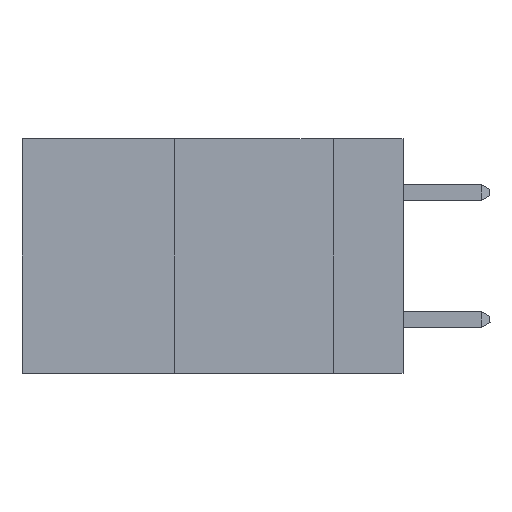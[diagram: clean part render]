
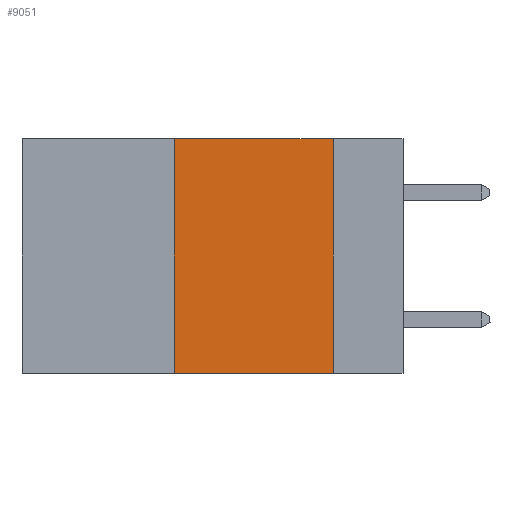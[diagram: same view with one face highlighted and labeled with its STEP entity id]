
A CAD part, left-side view. The second image highlights one B-rep face of the part: STEP entity #9051.
In plain terms, the highlighted planar face has unit normal (-1, 0, 0).
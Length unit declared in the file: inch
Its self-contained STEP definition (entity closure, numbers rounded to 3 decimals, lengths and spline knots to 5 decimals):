
#1376 = VERTEX_POINT ( 'NONE', #4658 ) ;
#2514 = CARTESIAN_POINT ( 'NONE',  ( 0., 0.6, -0.37 ) ) ;
#3719 = VERTEX_POINT ( 'NONE', #13797 ) ;
#4281 = ORIENTED_EDGE ( 'NONE', *, *, #21349, .T. ) ;
#4658 = CARTESIAN_POINT ( 'NONE',  ( 0., 0.11, -0.37 ) ) ;
#5012 = LINE ( 'NONE', #2514, #12658 ) ;
#5362 = ORIENTED_EDGE ( 'NONE', *, *, #29337, .F. ) ;
#7128 = CARTESIAN_POINT ( 'NONE',  ( 0., 0.11, 0. ) ) ;
#9051 = ADVANCED_FACE ( 'NONE', ( #9473 ), #32438, .F. ) ;
#9473 = FACE_OUTER_BOUND ( 'NONE', #40818, .T. ) ;
#10745 = LINE ( 'NONE', #16358, #35815 ) ;
#11396 = CARTESIAN_POINT ( 'NONE',  ( 0., 0.11, 0. ) ) ;
#12658 = VECTOR ( 'NONE', #22114, 39.37008 ) ;
#12799 = CARTESIAN_POINT ( 'NONE',  ( 0., 0.6, 0. ) ) ;
#13797 = CARTESIAN_POINT ( 'NONE',  ( 0., 0.36, 0. ) ) ;
#15226 = VECTOR ( 'NONE', #23618, 39.37008 ) ;
#16099 = DIRECTION ( 'NONE',  ( 1., 0., 0. ) ) ;
#16242 = LINE ( 'NONE', #7128, #15226 ) ;
#16358 = CARTESIAN_POINT ( 'NONE',  ( 0., 0.36, 0. ) ) ;
#17246 = EDGE_CURVE ( 'NONE', #3719, #19057, #24862, .T. ) ;
#17744 = CARTESIAN_POINT ( 'NONE',  ( 0., 0.36, -0.37 ) ) ;
#18602 = ORIENTED_EDGE ( 'NONE', *, *, #34459, .F. ) ;
#19057 = VERTEX_POINT ( 'NONE', #11396 ) ;
#21019 = VERTEX_POINT ( 'NONE', #17744 ) ;
#21349 = EDGE_CURVE ( 'NONE', #21019, #1376, #5012, .T. ) ;
#22114 = DIRECTION ( 'NONE',  ( 0., -1., 0. ) ) ;
#22837 = CARTESIAN_POINT ( 'NONE',  ( 0., 0.6, 0. ) ) ;
#23618 = DIRECTION ( 'NONE',  ( 0., 0., -1. ) ) ;
#24247 = ORIENTED_EDGE ( 'NONE', *, *, #17246, .F. ) ;
#24862 = LINE ( 'NONE', #22837, #40988 ) ;
#26143 = DIRECTION ( 'NONE',  ( 0., -1., 0. ) ) ;
#29337 = EDGE_CURVE ( 'NONE', #19057, #1376, #16242, .T. ) ;
#32438 = PLANE ( 'NONE',  #34838 ) ;
#32829 = DIRECTION ( 'NONE',  ( 0., 0., 1. ) ) ;
#34459 = EDGE_CURVE ( 'NONE', #21019, #3719, #10745, .T. ) ;
#34838 = AXIS2_PLACEMENT_3D ( 'NONE', #12799, #16099, #38848 ) ;
#35815 = VECTOR ( 'NONE', #32829, 39.37008 ) ;
#38848 = DIRECTION ( 'NONE',  ( 0., 0., -1. ) ) ;
#40818 = EDGE_LOOP ( 'NONE', ( #5362, #24247, #18602, #4281 ) ) ;
#40988 = VECTOR ( 'NONE', #26143, 39.37008 ) ;
